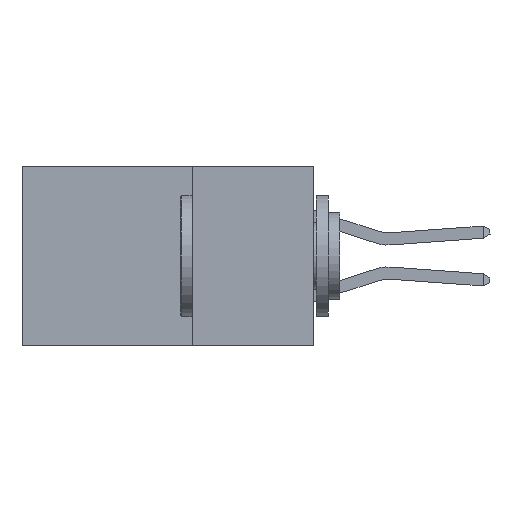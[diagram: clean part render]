
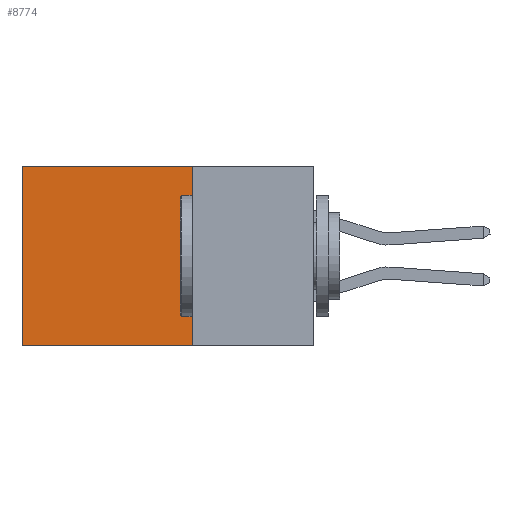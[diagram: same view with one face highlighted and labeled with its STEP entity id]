
A CAD part, left-side view. The second image highlights one B-rep face of the part: STEP entity #8774.
In plain terms, the highlighted planar face has unit normal (-1, 0, 0).
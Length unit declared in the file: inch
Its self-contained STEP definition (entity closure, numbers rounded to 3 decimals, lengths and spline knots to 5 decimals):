
#214 = EDGE_CURVE ( 'NONE', #1243, #1727, #5803, .T. ) ;
#547 = DIRECTION ( 'NONE',  ( 0., 0., -1. ) ) ;
#563 = VECTOR ( 'NONE', #16228, 39.37008 ) ;
#1063 = CARTESIAN_POINT ( 'NONE',  ( 0.2875, 0.6, 0. ) ) ;
#1243 = VERTEX_POINT ( 'NONE', #29945 ) ;
#1727 = VERTEX_POINT ( 'NONE', #1063 ) ;
#1946 = FACE_OUTER_BOUND ( 'NONE', #26718, .T. ) ;
#2479 = EDGE_CURVE ( 'NONE', #1243, #20746, #34297, .T. ) ;
#3142 = PLANE ( 'NONE',  #28058 ) ;
#3196 = VERTEX_POINT ( 'NONE', #33385 ) ;
#4437 = CARTESIAN_POINT ( 'NONE',  ( 0.2875, 0.25, -0.37 ) ) ;
#5803 = LINE ( 'NONE', #15013, #24866 ) ;
#7085 = LINE ( 'NONE', #4437, #10401 ) ;
#8774 = ADVANCED_FACE ( 'NONE', ( #1946 ), #3142, .F. ) ;
#10071 = DIRECTION ( 'NONE',  ( 0., 1., 0. ) ) ;
#10401 = VECTOR ( 'NONE', #31019, 39.37008 ) ;
#11630 = ORIENTED_EDGE ( 'NONE', *, *, #31135, .T. ) ;
#13810 = CARTESIAN_POINT ( 'NONE',  ( 0.2875, 0.6, 0. ) ) ;
#14059 = CARTESIAN_POINT ( 'NONE',  ( 0.2875, 0.25, 0. ) ) ;
#15013 = CARTESIAN_POINT ( 'NONE',  ( 0.2875, 0.25, 0. ) ) ;
#16228 = DIRECTION ( 'NONE',  ( 0., 0., -1. ) ) ;
#17753 = DIRECTION ( 'NONE',  ( 0., 0., -1. ) ) ;
#18702 = ORIENTED_EDGE ( 'NONE', *, *, #214, .T. ) ;
#19857 = ORIENTED_EDGE ( 'NONE', *, *, #2479, .F. ) ;
#20094 = VECTOR ( 'NONE', #17753, 39.37008 ) ;
#20746 = VERTEX_POINT ( 'NONE', #27521 ) ;
#22855 = ORIENTED_EDGE ( 'NONE', *, *, #33886, .F. ) ;
#24866 = VECTOR ( 'NONE', #10071, 39.37008 ) ;
#26718 = EDGE_LOOP ( 'NONE', ( #11630, #22855, #19857, #18702 ) ) ;
#27512 = DIRECTION ( 'NONE',  ( 1., 0., 0. ) ) ;
#27521 = CARTESIAN_POINT ( 'NONE',  ( 0.2875, 0.25, -0.37 ) ) ;
#28058 = AXIS2_PLACEMENT_3D ( 'NONE', #30101, #27512, #547 ) ;
#29945 = CARTESIAN_POINT ( 'NONE',  ( 0.2875, 0.25, 0. ) ) ;
#30101 = CARTESIAN_POINT ( 'NONE',  ( 0.2875, 0.25, 0. ) ) ;
#31019 = DIRECTION ( 'NONE',  ( 0., 1., 0. ) ) ;
#31135 = EDGE_CURVE ( 'NONE', #1727, #3196, #33395, .T. ) ;
#33385 = CARTESIAN_POINT ( 'NONE',  ( 0.2875, 0.6, -0.37 ) ) ;
#33395 = LINE ( 'NONE', #13810, #563 ) ;
#33886 = EDGE_CURVE ( 'NONE', #20746, #3196, #7085, .T. ) ;
#34297 = LINE ( 'NONE', #14059, #20094 ) ;
